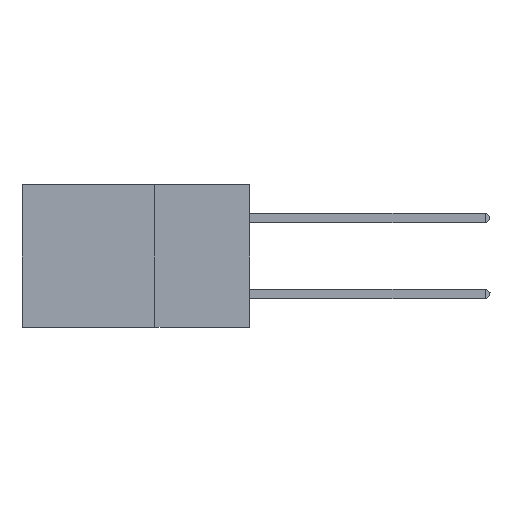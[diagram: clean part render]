
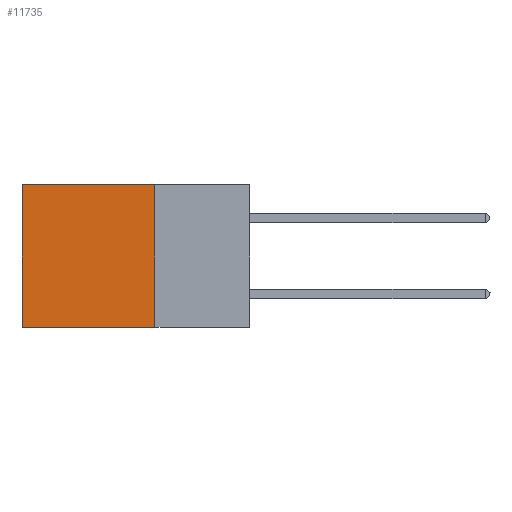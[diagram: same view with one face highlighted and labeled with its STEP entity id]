
A CAD part, left-side view. The second image highlights one B-rep face of the part: STEP entity #11735.
In plain terms, the highlighted planar face has unit normal (-1, 0, 0).
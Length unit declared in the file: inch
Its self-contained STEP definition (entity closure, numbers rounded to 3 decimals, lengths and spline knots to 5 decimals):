
#502 = EDGE_CURVE ( 'NONE', #971, #1417, #12250, .T. ) ;
#671 = DIRECTION ( 'NONE',  ( 0., 0., -1. ) ) ;
#878 = CARTESIAN_POINT ( 'NONE',  ( 0.2875, 0.25, 0. ) ) ;
#971 = VERTEX_POINT ( 'NONE', #878 ) ;
#1366 = FACE_OUTER_BOUND ( 'NONE', #13164, .T. ) ;
#1417 = VERTEX_POINT ( 'NONE', #7682 ) ;
#2370 = LINE ( 'NONE', #6220, #14906 ) ;
#3162 = VECTOR ( 'NONE', #671, 39.37008 ) ;
#3653 = EDGE_CURVE ( 'NONE', #971, #9079, #2370, .T. ) ;
#4442 = DIRECTION ( 'NONE',  ( 0., 1., 0. ) ) ;
#5020 = DIRECTION ( 'NONE',  ( 0., 0., -1. ) ) ;
#5560 = CARTESIAN_POINT ( 'NONE',  ( 0.2875, 0.6, -0.375 ) ) ;
#5887 = VECTOR ( 'NONE', #4442, 39.37008 ) ;
#6220 = CARTESIAN_POINT ( 'NONE',  ( 0.2875, 0.25, -0.375 ) ) ;
#6311 = PLANE ( 'NONE',  #9014 ) ;
#7529 = EDGE_CURVE ( 'NONE', #9079, #10109, #12010, .T. ) ;
#7610 = DIRECTION ( 'NONE',  ( 1., 0., 0. ) ) ;
#7682 = CARTESIAN_POINT ( 'NONE',  ( 0.2875, 0.6, 0. ) ) ;
#7795 = ORIENTED_EDGE ( 'NONE', *, *, #7529, .F. ) ;
#7972 = CARTESIAN_POINT ( 'NONE',  ( 0.2875, 0.25, -0.375 ) ) ;
#8032 = ORIENTED_EDGE ( 'NONE', *, *, #502, .T. ) ;
#8200 = DIRECTION ( 'NONE',  ( 0., 1., 0. ) ) ;
#8799 = CARTESIAN_POINT ( 'NONE',  ( 0.2875, 0.25, -0.375 ) ) ;
#8833 = CARTESIAN_POINT ( 'NONE',  ( 0.2875, 0.25, -0.375 ) ) ;
#9014 = AXIS2_PLACEMENT_3D ( 'NONE', #8833, #7610, #5020 ) ;
#9079 = VERTEX_POINT ( 'NONE', #8799 ) ;
#10025 = EDGE_CURVE ( 'NONE', #1417, #10109, #14005, .T. ) ;
#10109 = VERTEX_POINT ( 'NONE', #15229 ) ;
#11144 = DIRECTION ( 'NONE',  ( 0., 0., -1. ) ) ;
#11300 = ORIENTED_EDGE ( 'NONE', *, *, #3653, .F. ) ;
#11735 = ADVANCED_FACE ( 'NONE', ( #1366 ), #6311, .F. ) ;
#12010 = LINE ( 'NONE', #7972, #5887 ) ;
#12250 = LINE ( 'NONE', #15444, #13008 ) ;
#13008 = VECTOR ( 'NONE', #8200, 39.37008 ) ;
#13164 = EDGE_LOOP ( 'NONE', ( #14364, #7795, #11300, #8032 ) ) ;
#14005 = LINE ( 'NONE', #5560, #3162 ) ;
#14364 = ORIENTED_EDGE ( 'NONE', *, *, #10025, .T. ) ;
#14906 = VECTOR ( 'NONE', #11144, 39.37008 ) ;
#15229 = CARTESIAN_POINT ( 'NONE',  ( 0.2875, 0.6, -0.375 ) ) ;
#15444 = CARTESIAN_POINT ( 'NONE',  ( 0.2875, 0.25, 0. ) ) ;
